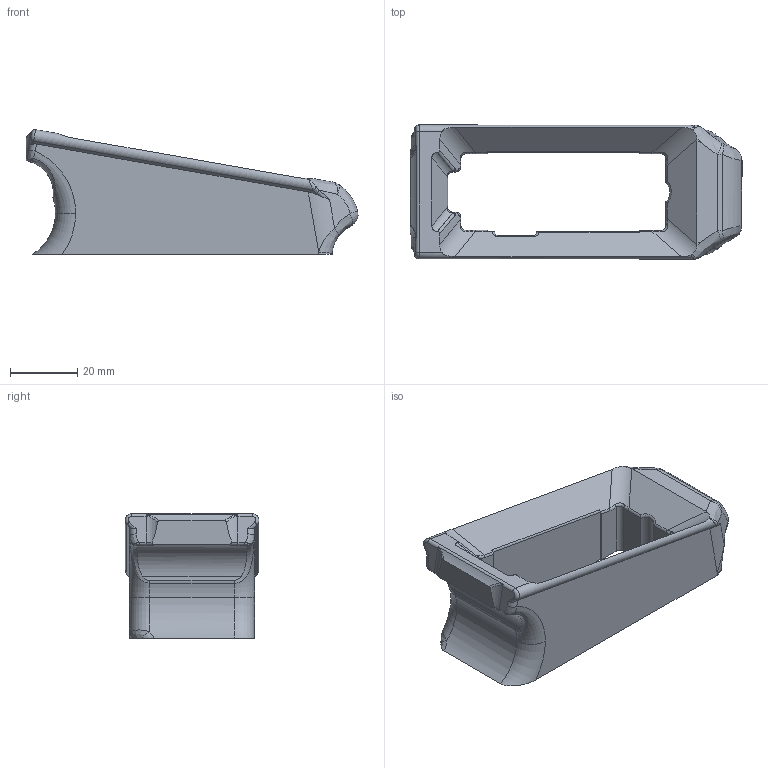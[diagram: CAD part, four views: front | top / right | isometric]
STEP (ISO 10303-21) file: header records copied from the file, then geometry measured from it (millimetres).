
FILE_DESCRIPTION (( 'STEP AP214' ), '1' );
FILE_NAME ('Magwell_3a.STEP', '2013-09-01T16:46:44', ( 'Asher' ), ( '' ), 'SwSTEP 2.0', 'SolidWorks 2013', '' );
FILE_SCHEMA (( 'AUTOMOTIVE_DESIGN' ));
Length unit declared in the file: millimetre
Products named in the file (1): Magwell_3a
Bounding box: 98.58 x 39.78 x 37.04 mm (x, y, z)
Volume: 44302.9 mm3; surface area: 15532.3 mm2
Topology: 1 solids, 1 shells, 190 faces, 483 edges, 289 vertices
Faces by surface type: bspline 64, cylinder 57, plane 51, torus 11, sphere 7
Entity records: 8384 total; most frequent: CARTESIAN_POINT 4417, ORIENTED_EDGE 956, DIRECTION 664, EDGE_CURVE 478, VERTEX_POINT 289, AXIS2_PLACEMENT_3D 242, EDGE_LOOP 191, ADVANCED_FACE 190
